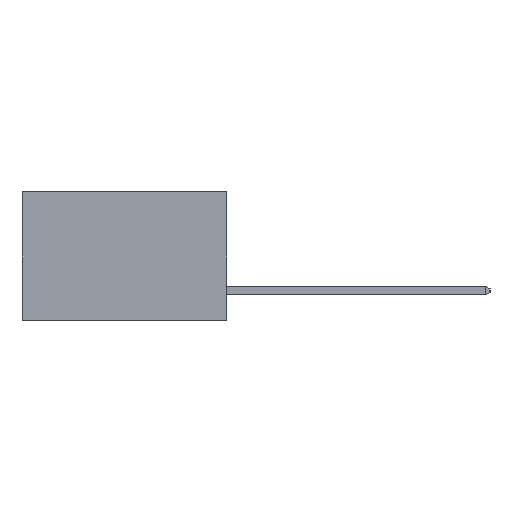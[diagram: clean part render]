
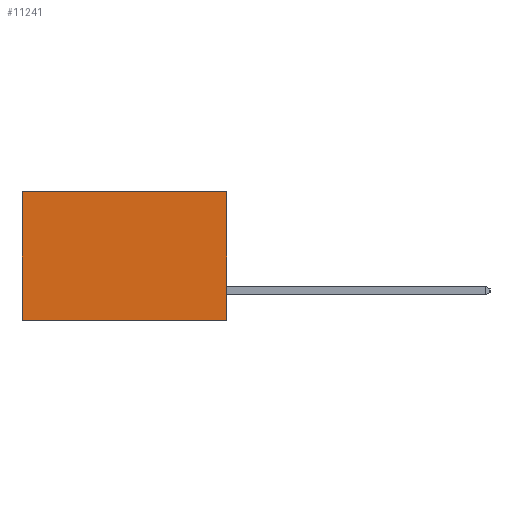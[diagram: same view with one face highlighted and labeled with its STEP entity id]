
A CAD part, left-side view. The second image highlights one B-rep face of the part: STEP entity #11241.
In plain terms, the highlighted planar face has unit normal (-1, 0, 0).
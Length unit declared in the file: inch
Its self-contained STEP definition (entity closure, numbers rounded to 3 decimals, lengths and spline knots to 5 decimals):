
#72 = EDGE_CURVE ( 'NONE', #5200, #943, #6924, .T. ) ;
#589 = DIRECTION ( 'NONE',  ( 0., 0., -1. ) ) ;
#607 = VERTEX_POINT ( 'NONE', #14440 ) ;
#943 = VERTEX_POINT ( 'NONE', #17066 ) ;
#1945 = EDGE_CURVE ( 'NONE', #5200, #607, #5937, .T. ) ;
#1998 = ORIENTED_EDGE ( 'NONE', *, *, #2077, .F. ) ;
#2040 = VECTOR ( 'NONE', #12907, 39.37008 ) ;
#2077 = EDGE_CURVE ( 'NONE', #943, #3726, #9509, .T. ) ;
#2275 = ORIENTED_EDGE ( 'NONE', *, *, #72, .F. ) ;
#3674 = PLANE ( 'NONE',  #17826 ) ;
#3726 = VERTEX_POINT ( 'NONE', #15780 ) ;
#4163 = DIRECTION ( 'NONE',  ( 0., 0., -1. ) ) ;
#5200 = VERTEX_POINT ( 'NONE', #13510 ) ;
#5702 = VECTOR ( 'NONE', #8506, 39.37008 ) ;
#5937 = LINE ( 'NONE', #10057, #2040 ) ;
#6038 = CARTESIAN_POINT ( 'NONE',  ( 0.277, 0., -0.37 ) ) ;
#6480 = VECTOR ( 'NONE', #4163, 39.37008 ) ;
#6591 = DIRECTION ( 'NONE',  ( 0., 0., -1. ) ) ;
#6924 = LINE ( 'NONE', #6038, #11196 ) ;
#6996 = CARTESIAN_POINT ( 'NONE',  ( 0.277, 0.59, -0.37 ) ) ;
#8506 = DIRECTION ( 'NONE',  ( 0., 1., 0. ) ) ;
#9509 = LINE ( 'NONE', #16563, #5702 ) ;
#10057 = CARTESIAN_POINT ( 'NONE',  ( 0.277, 0., 0. ) ) ;
#11180 = ORIENTED_EDGE ( 'NONE', *, *, #11854, .T. ) ;
#11196 = VECTOR ( 'NONE', #589, 39.37008 ) ;
#11241 = ADVANCED_FACE ( 'NONE', ( #13630 ), #3674, .F. ) ;
#11854 = EDGE_CURVE ( 'NONE', #607, #3726, #17656, .T. ) ;
#12907 = DIRECTION ( 'NONE',  ( 0., 1., 0. ) ) ;
#13510 = CARTESIAN_POINT ( 'NONE',  ( 0.277, 0., 0. ) ) ;
#13630 = FACE_OUTER_BOUND ( 'NONE', #17537, .T. ) ;
#13679 = CARTESIAN_POINT ( 'NONE',  ( 0.277, 0., -0.37 ) ) ;
#14440 = CARTESIAN_POINT ( 'NONE',  ( 0.277, 0.59, 0. ) ) ;
#15086 = DIRECTION ( 'NONE',  ( 1., 0., 0. ) ) ;
#15780 = CARTESIAN_POINT ( 'NONE',  ( 0.277, 0.59, -0.37 ) ) ;
#16563 = CARTESIAN_POINT ( 'NONE',  ( 0.277, 0., -0.37 ) ) ;
#17066 = CARTESIAN_POINT ( 'NONE',  ( 0.277, 0., -0.37 ) ) ;
#17109 = ORIENTED_EDGE ( 'NONE', *, *, #1945, .T. ) ;
#17537 = EDGE_LOOP ( 'NONE', ( #11180, #1998, #2275, #17109 ) ) ;
#17656 = LINE ( 'NONE', #6996, #6480 ) ;
#17826 = AXIS2_PLACEMENT_3D ( 'NONE', #13679, #15086, #6591 ) ;
